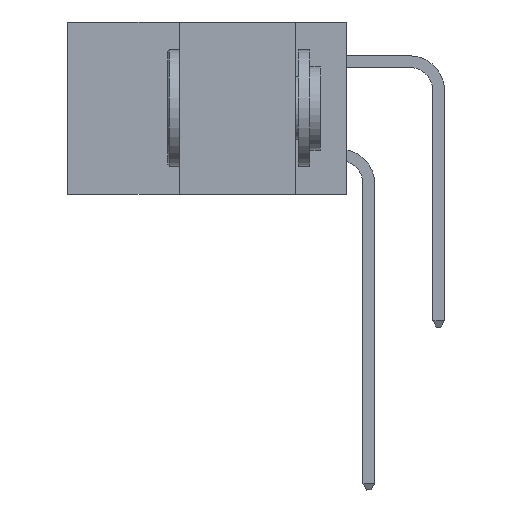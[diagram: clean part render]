
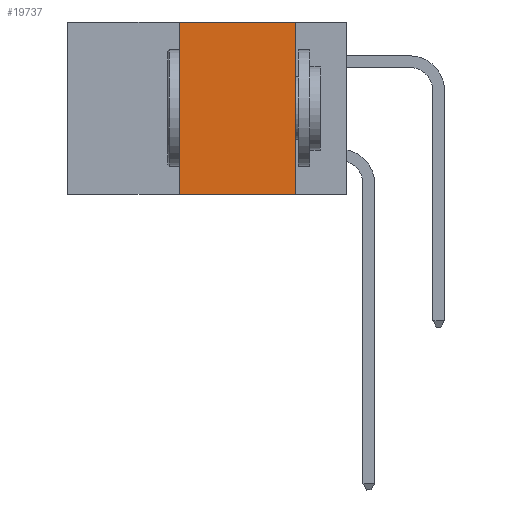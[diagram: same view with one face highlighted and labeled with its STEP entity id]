
A CAD part, left-side view. The second image highlights one B-rep face of the part: STEP entity #19737.
In plain terms, the highlighted planar face has unit normal (-1, 0, 0).
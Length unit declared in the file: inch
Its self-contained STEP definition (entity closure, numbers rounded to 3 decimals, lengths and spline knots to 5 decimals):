
#592 = VERTEX_POINT ( 'NONE', #6510 ) ;
#1739 = LINE ( 'NONE', #12080, #11094 ) ;
#2371 = EDGE_LOOP ( 'NONE', ( #6294, #8346, #7092, #22871 ) ) ;
#2540 = VECTOR ( 'NONE', #21560, 39.37008 ) ;
#2868 = AXIS2_PLACEMENT_3D ( 'NONE', #3292, #14480, #3370 ) ;
#3102 = LINE ( 'NONE', #19733, #2540 ) ;
#3292 = CARTESIAN_POINT ( 'NONE',  ( 0., 0.6, 0. ) ) ;
#3370 = DIRECTION ( 'NONE',  ( 0., 0., -1. ) ) ;
#3910 = CARTESIAN_POINT ( 'NONE',  ( 0., 0.11, 0. ) ) ;
#6294 = ORIENTED_EDGE ( 'NONE', *, *, #18896, .F. ) ;
#6510 = CARTESIAN_POINT ( 'NONE',  ( 0., 0.36, 0. ) ) ;
#6633 = EDGE_CURVE ( 'NONE', #10623, #9882, #1739, .T. ) ;
#7092 = ORIENTED_EDGE ( 'NONE', *, *, #15255, .F. ) ;
#8346 = ORIENTED_EDGE ( 'NONE', *, *, #9476, .F. ) ;
#9476 = EDGE_CURVE ( 'NONE', #592, #21689, #17669, .T. ) ;
#9882 = VERTEX_POINT ( 'NONE', #11184 ) ;
#10623 = VERTEX_POINT ( 'NONE', #18409 ) ;
#11094 = VECTOR ( 'NONE', #13909, 39.37008 ) ;
#11184 = CARTESIAN_POINT ( 'NONE',  ( 0., 0.11, -0.37 ) ) ;
#12068 = DIRECTION ( 'NONE',  ( 0., 0., -1. ) ) ;
#12080 = CARTESIAN_POINT ( 'NONE',  ( 0., 0.6, -0.37 ) ) ;
#13139 = FACE_OUTER_BOUND ( 'NONE', #2371, .T. ) ;
#13909 = DIRECTION ( 'NONE',  ( 0., -1., 0. ) ) ;
#14480 = DIRECTION ( 'NONE',  ( 1., 0., 0. ) ) ;
#15255 = EDGE_CURVE ( 'NONE', #10623, #592, #3102, .T. ) ;
#15601 = CARTESIAN_POINT ( 'NONE',  ( 0., 0.6, 0. ) ) ;
#17108 = VECTOR ( 'NONE', #17421, 39.37008 ) ;
#17421 = DIRECTION ( 'NONE',  ( 0., -1., 0. ) ) ;
#17669 = LINE ( 'NONE', #15601, #17108 ) ;
#18409 = CARTESIAN_POINT ( 'NONE',  ( 0., 0.36, -0.37 ) ) ;
#18896 = EDGE_CURVE ( 'NONE', #21689, #9882, #21057, .T. ) ;
#19733 = CARTESIAN_POINT ( 'NONE',  ( 0., 0.36, 0. ) ) ;
#19737 = ADVANCED_FACE ( 'NONE', ( #13139 ), #21641, .F. ) ;
#21057 = LINE ( 'NONE', #21064, #21610 ) ;
#21064 = CARTESIAN_POINT ( 'NONE',  ( 0., 0.11, 0. ) ) ;
#21560 = DIRECTION ( 'NONE',  ( 0., 0., 1. ) ) ;
#21610 = VECTOR ( 'NONE', #12068, 39.37008 ) ;
#21641 = PLANE ( 'NONE',  #2868 ) ;
#21689 = VERTEX_POINT ( 'NONE', #3910 ) ;
#22871 = ORIENTED_EDGE ( 'NONE', *, *, #6633, .T. ) ;
